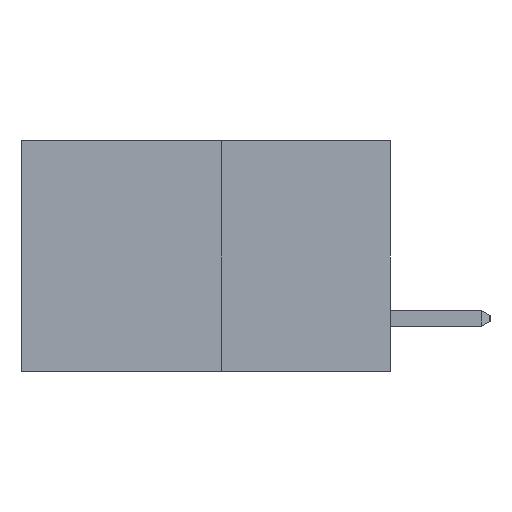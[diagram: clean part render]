
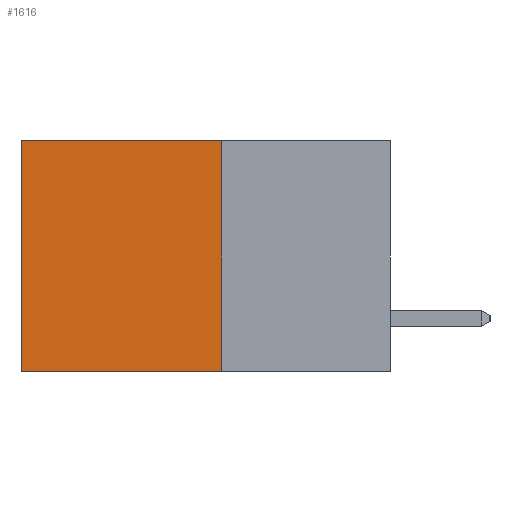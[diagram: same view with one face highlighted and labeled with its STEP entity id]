
A CAD part, left-side view. The second image highlights one B-rep face of the part: STEP entity #1616.
In plain terms, the highlighted planar face has unit normal (-1, 0, 0).
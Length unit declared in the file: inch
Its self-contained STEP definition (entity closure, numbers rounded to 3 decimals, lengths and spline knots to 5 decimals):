
#80 = LINE ( 'NONE', #7273, #2359 ) ;
#128 = PLANE ( 'NONE',  #9023 ) ;
#367 = CARTESIAN_POINT ( 'NONE',  ( 0.277, 0.27, 0. ) ) ;
#430 = DIRECTION ( 'NONE',  ( 0., 1., 0. ) ) ;
#520 = VERTEX_POINT ( 'NONE', #1779 ) ;
#651 = CARTESIAN_POINT ( 'NONE',  ( 0.277, 0.27, 0. ) ) ;
#948 = VECTOR ( 'NONE', #2606, 39.37008 ) ;
#1347 = EDGE_CURVE ( 'NONE', #1725, #4782, #4030, .T. ) ;
#1350 = ORIENTED_EDGE ( 'NONE', *, *, #2902, .F. ) ;
#1473 = EDGE_LOOP ( 'NONE', ( #4660, #1780, #1350, #1596 ) ) ;
#1596 = ORIENTED_EDGE ( 'NONE', *, *, #1347, .T. ) ;
#1616 = ADVANCED_FACE ( 'NONE', ( #4730 ), #128, .F. ) ;
#1696 = VECTOR ( 'NONE', #430, 39.37008 ) ;
#1725 = VERTEX_POINT ( 'NONE', #651 ) ;
#1779 = CARTESIAN_POINT ( 'NONE',  ( 0.277, 0.27, -0.37 ) ) ;
#1780 = ORIENTED_EDGE ( 'NONE', *, *, #8448, .F. ) ;
#1933 = CARTESIAN_POINT ( 'NONE',  ( 0.277, 0.27, -0.37 ) ) ;
#2359 = VECTOR ( 'NONE', #4597, 39.37008 ) ;
#2606 = DIRECTION ( 'NONE',  ( 0., 0., -1. ) ) ;
#2902 = EDGE_CURVE ( 'NONE', #1725, #520, #7163, .T. ) ;
#3532 = VERTEX_POINT ( 'NONE', #3666 ) ;
#3666 = CARTESIAN_POINT ( 'NONE',  ( 0.277, 0.59, -0.37 ) ) ;
#4030 = LINE ( 'NONE', #367, #1696 ) ;
#4134 = LINE ( 'NONE', #1933, #7770 ) ;
#4564 = DIRECTION ( 'NONE',  ( 0., 0., -1. ) ) ;
#4577 = DIRECTION ( 'NONE',  ( 1., 0., 0. ) ) ;
#4597 = DIRECTION ( 'NONE',  ( 0., 0., -1. ) ) ;
#4660 = ORIENTED_EDGE ( 'NONE', *, *, #6588, .T. ) ;
#4730 = FACE_OUTER_BOUND ( 'NONE', #1473, .T. ) ;
#4782 = VERTEX_POINT ( 'NONE', #9006 ) ;
#6588 = EDGE_CURVE ( 'NONE', #4782, #3532, #80, .T. ) ;
#6718 = CARTESIAN_POINT ( 'NONE',  ( 0.277, 0.27, -0.37 ) ) ;
#7163 = LINE ( 'NONE', #6718, #948 ) ;
#7273 = CARTESIAN_POINT ( 'NONE',  ( 0.277, 0.59, -0.37 ) ) ;
#7770 = VECTOR ( 'NONE', #8027, 39.37008 ) ;
#8027 = DIRECTION ( 'NONE',  ( 0., 1., 0. ) ) ;
#8137 = CARTESIAN_POINT ( 'NONE',  ( 0.277, 0.27, -0.37 ) ) ;
#8448 = EDGE_CURVE ( 'NONE', #520, #3532, #4134, .T. ) ;
#9006 = CARTESIAN_POINT ( 'NONE',  ( 0.277, 0.59, 0. ) ) ;
#9023 = AXIS2_PLACEMENT_3D ( 'NONE', #8137, #4577, #4564 ) ;
